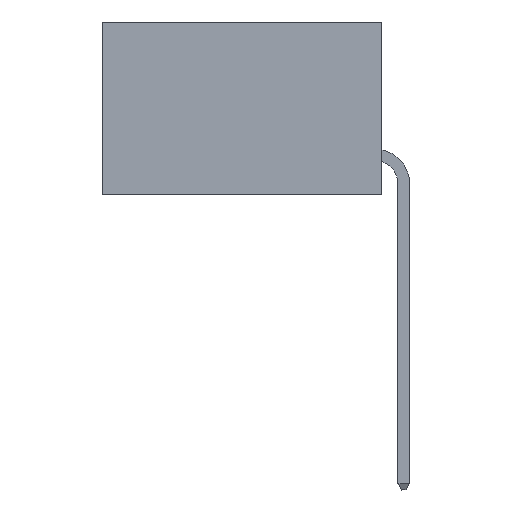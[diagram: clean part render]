
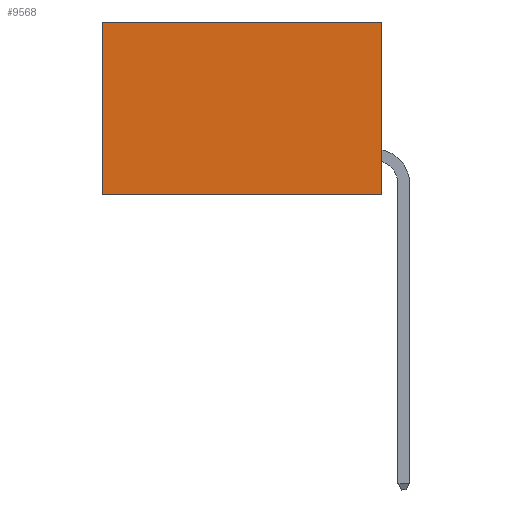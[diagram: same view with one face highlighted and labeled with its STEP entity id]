
A CAD part, left-side view. The second image highlights one B-rep face of the part: STEP entity #9568.
In plain terms, the highlighted planar face has unit normal (-1, 0, 0).
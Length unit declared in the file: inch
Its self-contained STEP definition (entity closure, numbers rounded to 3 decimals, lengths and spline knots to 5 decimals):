
#1647 = EDGE_CURVE ( 'NONE', #12058, #40568, #34996, .T. ) ;
#1919 = EDGE_CURVE ( 'NONE', #43261, #40568, #8027, .T. ) ;
#2619 = CARTESIAN_POINT ( 'NONE',  ( 0.2875, 0., 0. ) ) ;
#3033 = CARTESIAN_POINT ( 'NONE',  ( 0.2875, 0., 0. ) ) ;
#5531 = EDGE_CURVE ( 'NONE', #23808, #12058, #38342, .T. ) ;
#5840 = CARTESIAN_POINT ( 'NONE',  ( 0.2875, 0., 0. ) ) ;
#6362 = VECTOR ( 'NONE', #20871, 39.37008 ) ;
#8027 = LINE ( 'NONE', #40567, #40822 ) ;
#9164 = CARTESIAN_POINT ( 'NONE',  ( 0.2875, 0.6, 0. ) ) ;
#9568 = ADVANCED_FACE ( 'NONE', ( #32700 ), #16094, .F. ) ;
#12058 = VERTEX_POINT ( 'NONE', #39602 ) ;
#16094 = PLANE ( 'NONE',  #30896 ) ;
#17885 = ORIENTED_EDGE ( 'NONE', *, *, #1647, .T. ) ;
#19660 = DIRECTION ( 'NONE',  ( 0., 0., -1. ) ) ;
#19820 = DIRECTION ( 'NONE',  ( 0., 1., 0. ) ) ;
#19868 = EDGE_CURVE ( 'NONE', #23808, #43261, #27449, .T. ) ;
#20871 = DIRECTION ( 'NONE',  ( 0., 0., -1. ) ) ;
#22042 = ORIENTED_EDGE ( 'NONE', *, *, #5531, .T. ) ;
#22396 = VECTOR ( 'NONE', #40064, 39.37008 ) ;
#22414 = ORIENTED_EDGE ( 'NONE', *, *, #1919, .F. ) ;
#23808 = VERTEX_POINT ( 'NONE', #36086 ) ;
#23962 = EDGE_LOOP ( 'NONE', ( #17885, #22414, #34881, #22042 ) ) ;
#25799 = DIRECTION ( 'NONE',  ( 0., 1., 0. ) ) ;
#27449 = LINE ( 'NONE', #3033, #6362 ) ;
#29476 = CARTESIAN_POINT ( 'NONE',  ( 0.2875, 0.6, -0.37 ) ) ;
#30896 = AXIS2_PLACEMENT_3D ( 'NONE', #2619, #39874, #19660 ) ;
#32583 = CARTESIAN_POINT ( 'NONE',  ( 0.2875, 0., -0.37 ) ) ;
#32700 = FACE_OUTER_BOUND ( 'NONE', #23962, .T. ) ;
#34881 = ORIENTED_EDGE ( 'NONE', *, *, #19868, .F. ) ;
#34996 = LINE ( 'NONE', #9164, #22396 ) ;
#35752 = VECTOR ( 'NONE', #25799, 39.37008 ) ;
#36086 = CARTESIAN_POINT ( 'NONE',  ( 0.2875, 0., 0. ) ) ;
#38342 = LINE ( 'NONE', #5840, #35752 ) ;
#39602 = CARTESIAN_POINT ( 'NONE',  ( 0.2875, 0.6, 0. ) ) ;
#39874 = DIRECTION ( 'NONE',  ( 1., 0., 0. ) ) ;
#40064 = DIRECTION ( 'NONE',  ( 0., 0., -1. ) ) ;
#40567 = CARTESIAN_POINT ( 'NONE',  ( 0.2875, 0., -0.37 ) ) ;
#40568 = VERTEX_POINT ( 'NONE', #29476 ) ;
#40822 = VECTOR ( 'NONE', #19820, 39.37008 ) ;
#43261 = VERTEX_POINT ( 'NONE', #32583 ) ;
